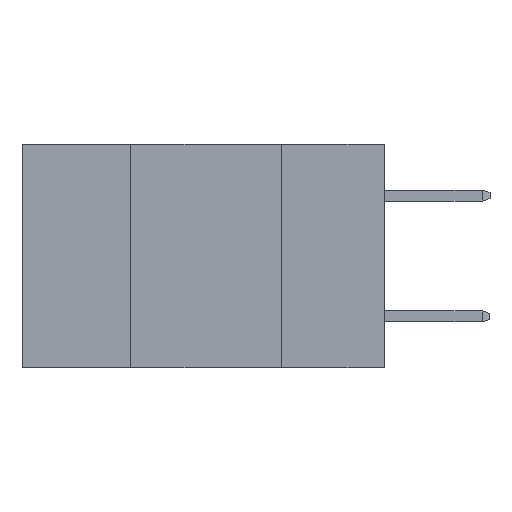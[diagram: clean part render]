
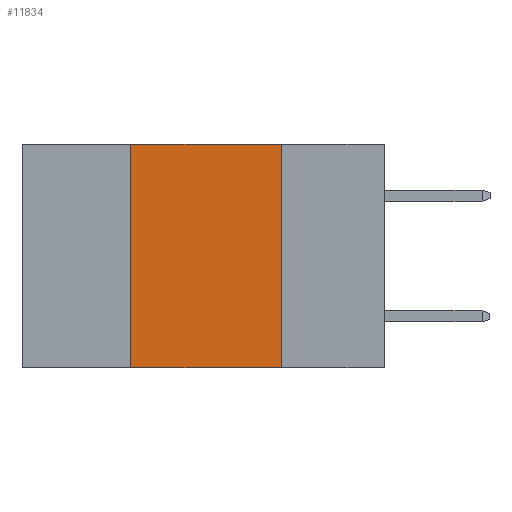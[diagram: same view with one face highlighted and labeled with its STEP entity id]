
A CAD part, left-side view. The second image highlights one B-rep face of the part: STEP entity #11834.
In plain terms, the highlighted planar face has unit normal (-1, 0, 0).
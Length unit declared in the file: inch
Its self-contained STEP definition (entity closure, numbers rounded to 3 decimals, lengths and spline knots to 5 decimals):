
#930 = CARTESIAN_POINT ( 'NONE',  ( 0., 0.17, -0.37 ) ) ;
#994 = CARTESIAN_POINT ( 'NONE',  ( 0., 0.6, 0. ) ) ;
#1422 = VERTEX_POINT ( 'NONE', #3369 ) ;
#1471 = EDGE_LOOP ( 'NONE', ( #4729, #9689, #9817, #3603 ) ) ;
#1556 = CARTESIAN_POINT ( 'NONE',  ( 0., 0.6, 0. ) ) ;
#1884 = VECTOR ( 'NONE', #4430, 39.37008 ) ;
#2019 = DIRECTION ( 'NONE',  ( 0., 0., -1. ) ) ;
#2191 = LINE ( 'NONE', #7161, #1884 ) ;
#2251 = CARTESIAN_POINT ( 'NONE',  ( 0., 0.42, 0. ) ) ;
#2771 = AXIS2_PLACEMENT_3D ( 'NONE', #994, #7529, #2019 ) ;
#2787 = LINE ( 'NONE', #10540, #4686 ) ;
#2800 = CARTESIAN_POINT ( 'NONE',  ( 0., 0.42, 0. ) ) ;
#3183 = DIRECTION ( 'NONE',  ( 0., 0., 1. ) ) ;
#3369 = CARTESIAN_POINT ( 'NONE',  ( 0., 0.42, -0.37 ) ) ;
#3465 = DIRECTION ( 'NONE',  ( 0., -1., 0. ) ) ;
#3493 = VECTOR ( 'NONE', #3183, 39.37008 ) ;
#3603 = ORIENTED_EDGE ( 'NONE', *, *, #6094, .T. ) ;
#3747 = VERTEX_POINT ( 'NONE', #2800 ) ;
#4183 = EDGE_CURVE ( 'NONE', #3747, #8147, #10959, .T. ) ;
#4430 = DIRECTION ( 'NONE',  ( 0., -1., 0. ) ) ;
#4686 = VECTOR ( 'NONE', #11454, 39.37008 ) ;
#4722 = EDGE_CURVE ( 'NONE', #8147, #6985, #2787, .T. ) ;
#4729 = ORIENTED_EDGE ( 'NONE', *, *, #4722, .F. ) ;
#4772 = PLANE ( 'NONE',  #2771 ) ;
#5201 = FACE_OUTER_BOUND ( 'NONE', #1471, .T. ) ;
#5569 = VECTOR ( 'NONE', #3465, 39.37008 ) ;
#5969 = LINE ( 'NONE', #2251, #3493 ) ;
#6094 = EDGE_CURVE ( 'NONE', #1422, #6985, #2191, .T. ) ;
#6436 = CARTESIAN_POINT ( 'NONE',  ( 0., 0.17, 0. ) ) ;
#6985 = VERTEX_POINT ( 'NONE', #930 ) ;
#7161 = CARTESIAN_POINT ( 'NONE',  ( 0., 0.6, -0.37 ) ) ;
#7529 = DIRECTION ( 'NONE',  ( 1., 0., 0. ) ) ;
#8147 = VERTEX_POINT ( 'NONE', #6436 ) ;
#9689 = ORIENTED_EDGE ( 'NONE', *, *, #4183, .F. ) ;
#9817 = ORIENTED_EDGE ( 'NONE', *, *, #10722, .F. ) ;
#10540 = CARTESIAN_POINT ( 'NONE',  ( 0., 0.17, 0. ) ) ;
#10722 = EDGE_CURVE ( 'NONE', #1422, #3747, #5969, .T. ) ;
#10959 = LINE ( 'NONE', #1556, #5569 ) ;
#11454 = DIRECTION ( 'NONE',  ( 0., 0., -1. ) ) ;
#11834 = ADVANCED_FACE ( 'NONE', ( #5201 ), #4772, .F. ) ;
